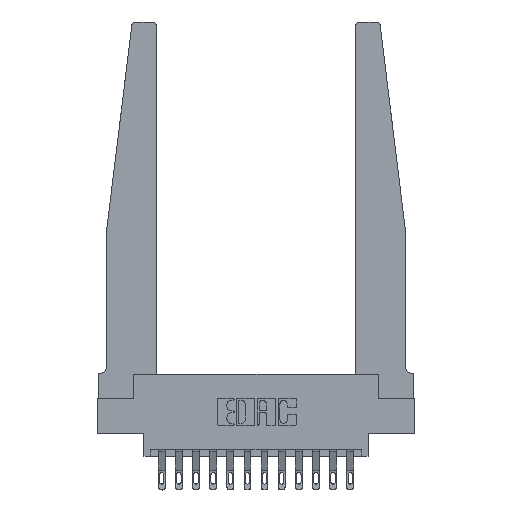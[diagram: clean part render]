
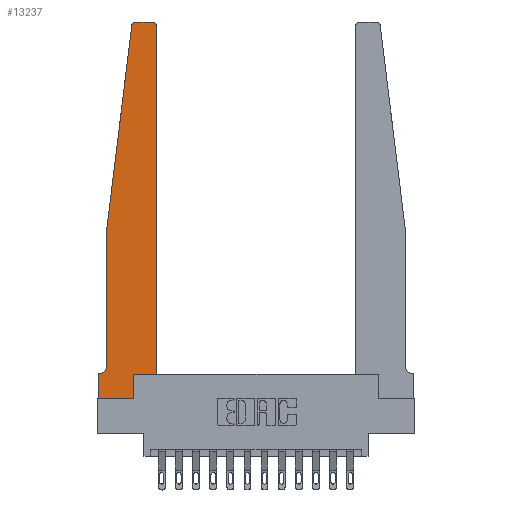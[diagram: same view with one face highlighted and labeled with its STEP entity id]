
A CAD part, top view. The second image highlights one B-rep face of the part: STEP entity #13237.
In plain terms, the highlighted planar face has unit normal (0, 0, 1).
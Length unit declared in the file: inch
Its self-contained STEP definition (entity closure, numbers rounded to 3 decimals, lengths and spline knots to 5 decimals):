
#225 = EDGE_CURVE ( 'NONE', #10030, #5206, #12877, .T. ) ;
#420 = CARTESIAN_POINT ( 'NONE',  ( 0., 0., 0.37 ) ) ;
#496 = VECTOR ( 'NONE', #2696, 39.37008 ) ;
#591 = CIRCLE ( 'NONE', #9966, 0.05 ) ;
#755 = EDGE_LOOP ( 'NONE', ( #10475, #10082, #8857, #10367, #7473, #12838, #9328, #15527, #16552, #3514, #12187, #2093 ) ) ;
#1061 = VECTOR ( 'NONE', #6143, 39.37008 ) ;
#1206 = VERTEX_POINT ( 'NONE', #13017 ) ;
#1706 = VECTOR ( 'NONE', #15763, 39.37008 ) ;
#1746 = CARTESIAN_POINT ( 'NONE',  ( 0., 0.1875, 0.37 ) ) ;
#1970 = DIRECTION ( 'NONE',  ( -1., 0., 0. ) ) ;
#2053 = DIRECTION ( 'NONE',  ( 0., 0., 1. ) ) ;
#2093 = ORIENTED_EDGE ( 'NONE', *, *, #7554, .T. ) ;
#2296 = CARTESIAN_POINT ( 'NONE',  ( 0.27653, 2.72, 0.37 ) ) ;
#2314 = CARTESIAN_POINT ( 'NONE',  ( 0.065, 1.25, 0.37 ) ) ;
#2362 = VECTOR ( 'NONE', #15619, 39.37008 ) ;
#2391 = CARTESIAN_POINT ( 'NONE',  ( 0., 0., 0.37 ) ) ;
#2696 = DIRECTION ( 'NONE',  ( -1., 0., 0. ) ) ;
#3032 = VECTOR ( 'NONE', #10994, 39.37008 ) ;
#3099 = CARTESIAN_POINT ( 'NONE',  ( 0.425, 0.18, 0.37 ) ) ;
#3220 = CARTESIAN_POINT ( 'NONE',  ( 0.015, 0.2375, 0.37 ) ) ;
#3514 = ORIENTED_EDGE ( 'NONE', *, *, #4044, .T. ) ;
#3625 = DIRECTION ( 'NONE',  ( 1., 0., 0. ) ) ;
#3732 = EDGE_CURVE ( 'NONE', #9495, #10030, #6681, .T. ) ;
#3968 = CARTESIAN_POINT ( 'NONE',  ( 0.25, 2.75, 0.37 ) ) ;
#4038 = LINE ( 'NONE', #3968, #496 ) ;
#4044 = EDGE_CURVE ( 'NONE', #5051, #7390, #15767, .T. ) ;
#4361 = VERTEX_POINT ( 'NONE', #8497 ) ;
#4511 = VERTEX_POINT ( 'NONE', #8792 ) ;
#4560 = DIRECTION ( 'NONE',  ( -1., 0., 0. ) ) ;
#4618 = CARTESIAN_POINT ( 'NONE',  ( 0.065, 0.1875, 0.37 ) ) ;
#4856 = CARTESIAN_POINT ( 'NONE',  ( 0.27653, 2.75, 0.37 ) ) ;
#5051 = VERTEX_POINT ( 'NONE', #8537 ) ;
#5187 = VERTEX_POINT ( 'NONE', #4856 ) ;
#5206 = VERTEX_POINT ( 'NONE', #7498 ) ;
#5436 = VECTOR ( 'NONE', #15451, 39.37008 ) ;
#5597 = VECTOR ( 'NONE', #10192, 39.37008 ) ;
#5839 = LINE ( 'NONE', #8861, #5436 ) ;
#5874 = DIRECTION ( 'NONE',  ( 0., 1., 0. ) ) ;
#5979 = EDGE_CURVE ( 'NONE', #4511, #9495, #591, .T. ) ;
#6143 = DIRECTION ( 'NONE',  ( 0., -1., 0. ) ) ;
#6639 = CARTESIAN_POINT ( 'NONE',  ( 0.395, 2.72, 0.37 ) ) ;
#6681 = LINE ( 'NONE', #4618, #9752 ) ;
#6789 = VERTEX_POINT ( 'NONE', #12769 ) ;
#7285 = PLANE ( 'NONE',  #13672 ) ;
#7390 = VERTEX_POINT ( 'NONE', #10083 ) ;
#7395 = VERTEX_POINT ( 'NONE', #16697 ) ;
#7473 = ORIENTED_EDGE ( 'NONE', *, *, #5979, .T. ) ;
#7498 = CARTESIAN_POINT ( 'NONE',  ( 0., 0., 0.37 ) ) ;
#7554 = EDGE_CURVE ( 'NONE', #4361, #16264, #14628, .T. ) ;
#7815 = CARTESIAN_POINT ( 'NONE',  ( 0.425, 0.18, 0.37 ) ) ;
#7944 = DIRECTION ( 'NONE',  ( 1., 0., 0. ) ) ;
#8069 = LINE ( 'NONE', #11382, #1061 ) ;
#8283 = EDGE_CURVE ( 'NONE', #5206, #7395, #10457, .T. ) ;
#8317 = AXIS2_PLACEMENT_3D ( 'NONE', #6639, #15889, #7944 ) ;
#8497 = CARTESIAN_POINT ( 'NONE',  ( 0.425, 2.72, 0.37 ) ) ;
#8537 = CARTESIAN_POINT ( 'NONE',  ( 0.2605, 0.18, 0.37 ) ) ;
#8604 = CARTESIAN_POINT ( 'NONE',  ( 0., 0.1875, 0.37 ) ) ;
#8608 = AXIS2_PLACEMENT_3D ( 'NONE', #2296, #11535, #3625 ) ;
#8792 = CARTESIAN_POINT ( 'NONE',  ( 0.065, 0.2375, 0.37 ) ) ;
#8857 = ORIENTED_EDGE ( 'NONE', *, *, #13982, .T. ) ;
#8861 = CARTESIAN_POINT ( 'NONE',  ( 0.2605, 0.18, 0.37 ) ) ;
#9058 = EDGE_CURVE ( 'NONE', #7390, #4361, #10211, .T. ) ;
#9328 = ORIENTED_EDGE ( 'NONE', *, *, #225, .T. ) ;
#9472 = EDGE_CURVE ( 'NONE', #16264, #5187, #4038, .T. ) ;
#9495 = VERTEX_POINT ( 'NONE', #10645 ) ;
#9752 = VECTOR ( 'NONE', #1970, 39.37008 ) ;
#9966 = AXIS2_PLACEMENT_3D ( 'NONE', #3220, #12446, #4560 ) ;
#10030 = VERTEX_POINT ( 'NONE', #1746 ) ;
#10082 = ORIENTED_EDGE ( 'NONE', *, *, #16327, .T. ) ;
#10083 = CARTESIAN_POINT ( 'NONE',  ( 0.425, 0.18, 0.37 ) ) ;
#10192 = DIRECTION ( 'NONE',  ( -0.122, -0.992, 0. ) ) ;
#10211 = LINE ( 'NONE', #3099, #13741 ) ;
#10367 = ORIENTED_EDGE ( 'NONE', *, *, #13317, .T. ) ;
#10457 = LINE ( 'NONE', #420, #3032 ) ;
#10475 = ORIENTED_EDGE ( 'NONE', *, *, #9472, .T. ) ;
#10645 = CARTESIAN_POINT ( 'NONE',  ( 0.015, 0.1875, 0.37 ) ) ;
#10994 = DIRECTION ( 'NONE',  ( 1., 0., 0. ) ) ;
#11278 = DIRECTION ( 'NONE',  ( 1., 0., 0. ) ) ;
#11382 = CARTESIAN_POINT ( 'NONE',  ( 0.065, 1.25, 0.37 ) ) ;
#11535 = DIRECTION ( 'NONE',  ( 0., 0., 1. ) ) ;
#12187 = ORIENTED_EDGE ( 'NONE', *, *, #9058, .T. ) ;
#12421 = FACE_OUTER_BOUND ( 'NONE', #755, .T. ) ;
#12446 = DIRECTION ( 'NONE',  ( 0., 0., -1. ) ) ;
#12756 = EDGE_CURVE ( 'NONE', #7395, #5051, #5839, .T. ) ;
#12769 = CARTESIAN_POINT ( 'NONE',  ( 0.065, 1.25, 0.37 ) ) ;
#12838 = ORIENTED_EDGE ( 'NONE', *, *, #3732, .T. ) ;
#12877 = LINE ( 'NONE', #2391, #2362 ) ;
#13015 = LINE ( 'NONE', #2314, #5597 ) ;
#13017 = CARTESIAN_POINT ( 'NONE',  ( 0.24675, 2.72367, 0.37 ) ) ;
#13237 = ADVANCED_FACE ( 'NONE', ( #12421 ), #7285, .T. ) ;
#13317 = EDGE_CURVE ( 'NONE', #6789, #4511, #8069, .T. ) ;
#13672 = AXIS2_PLACEMENT_3D ( 'NONE', #8604, #2053, #11278 ) ;
#13741 = VECTOR ( 'NONE', #5874, 39.37008 ) ;
#13982 = EDGE_CURVE ( 'NONE', #1206, #6789, #13015, .T. ) ;
#14014 = CARTESIAN_POINT ( 'NONE',  ( 0.395, 2.75, 0.37 ) ) ;
#14628 = CIRCLE ( 'NONE', #8317, 0.03 ) ;
#15435 = CIRCLE ( 'NONE', #8608, 0.03 ) ;
#15451 = DIRECTION ( 'NONE',  ( 0., 1., 0. ) ) ;
#15527 = ORIENTED_EDGE ( 'NONE', *, *, #8283, .T. ) ;
#15619 = DIRECTION ( 'NONE',  ( 0., -1., 0. ) ) ;
#15763 = DIRECTION ( 'NONE',  ( 1., 0., 0. ) ) ;
#15767 = LINE ( 'NONE', #7815, #1706 ) ;
#15889 = DIRECTION ( 'NONE',  ( 0., 0., 1. ) ) ;
#16264 = VERTEX_POINT ( 'NONE', #14014 ) ;
#16327 = EDGE_CURVE ( 'NONE', #5187, #1206, #15435, .T. ) ;
#16552 = ORIENTED_EDGE ( 'NONE', *, *, #12756, .T. ) ;
#16697 = CARTESIAN_POINT ( 'NONE',  ( 0.2605, 0., 0.37 ) ) ;
